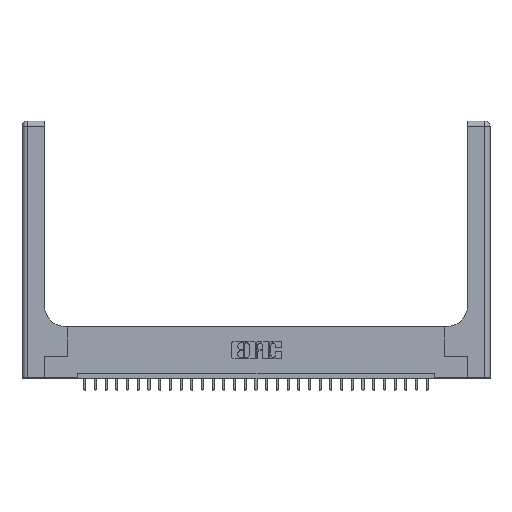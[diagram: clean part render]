
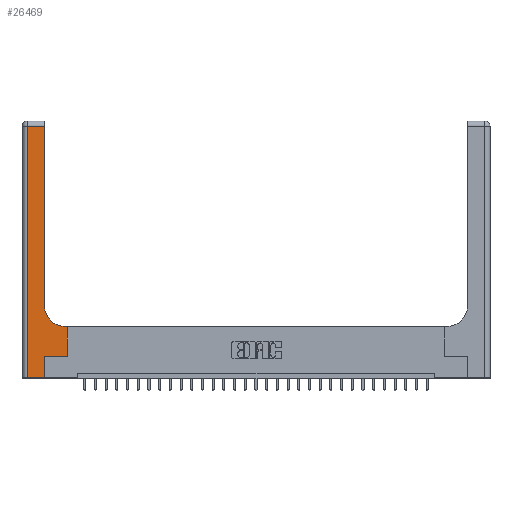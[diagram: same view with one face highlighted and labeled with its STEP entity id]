
A CAD part, top view. The second image highlights one B-rep face of the part: STEP entity #26469.
In plain terms, the highlighted planar face has unit normal (0, 0, 1).
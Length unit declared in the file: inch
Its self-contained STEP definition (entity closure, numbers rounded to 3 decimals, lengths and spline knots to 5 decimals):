
#18 = EDGE_LOOP ( 'NONE', ( #2493, #15372, #7618, #73, #6283, #25855, #7352, #18004, #8994 ) ) ;
#73 = ORIENTED_EDGE ( 'NONE', *, *, #17426, .T. ) ;
#368 = LINE ( 'NONE', #19405, #23107 ) ;
#612 = VERTEX_POINT ( 'NONE', #10977 ) ;
#644 = VECTOR ( 'NONE', #1093, 39.37008 ) ;
#657 = VECTOR ( 'NONE', #3164, 39.37008 ) ;
#1093 = DIRECTION ( 'NONE',  ( 1., 0., 0. ) ) ;
#1325 = CARTESIAN_POINT ( 'NONE',  ( 0.265, 0., 0.37 ) ) ;
#1657 = VERTEX_POINT ( 'NONE', #12036 ) ;
#1805 = VERTEX_POINT ( 'NONE', #18452 ) ;
#1813 = DIRECTION ( 'NONE',  ( 1., 0., 0. ) ) ;
#2021 = EDGE_CURVE ( 'NONE', #4811, #21082, #368, .T. ) ;
#2050 = VECTOR ( 'NONE', #3155, 39.37008 ) ;
#2493 = ORIENTED_EDGE ( 'NONE', *, *, #2021, .T. ) ;
#2524 = CARTESIAN_POINT ( 'NONE',  ( 0., 2.94, 0.37 ) ) ;
#3155 = DIRECTION ( 'NONE',  ( 1., 0., 0. ) ) ;
#3164 = DIRECTION ( 'NONE',  ( 0., 1., 0. ) ) ;
#3475 = EDGE_CURVE ( 'NONE', #21082, #24802, #25972, .T. ) ;
#3976 = CARTESIAN_POINT ( 'NONE',  ( 0.06, 3., 0.37 ) ) ;
#4811 = VERTEX_POINT ( 'NONE', #6078 ) ;
#4902 = EDGE_CURVE ( 'NONE', #612, #4811, #15092, .T. ) ;
#5114 = CARTESIAN_POINT ( 'NONE',  ( 0.265, 0.25, 0.37 ) ) ;
#5139 = DIRECTION ( 'NONE',  ( 0., 1., 0. ) ) ;
#5498 = DIRECTION ( 'NONE',  ( -1., 0., 0. ) ) ;
#5923 = CARTESIAN_POINT ( 'NONE',  ( 0.51, 0.85, 0.37 ) ) ;
#5949 = FACE_OUTER_BOUND ( 'NONE', #18, .T. ) ;
#6078 = CARTESIAN_POINT ( 'NONE',  ( 0.26, 0.85, 0.37 ) ) ;
#6159 = CARTESIAN_POINT ( 'NONE',  ( 0.26, 2.94, 0.37 ) ) ;
#6283 = ORIENTED_EDGE ( 'NONE', *, *, #12287, .T. ) ;
#7228 = EDGE_CURVE ( 'NONE', #22148, #25011, #16596, .T. ) ;
#7295 = VERTEX_POINT ( 'NONE', #7666 ) ;
#7352 = ORIENTED_EDGE ( 'NONE', *, *, #18931, .T. ) ;
#7447 = LINE ( 'NONE', #26327, #15210 ) ;
#7618 = ORIENTED_EDGE ( 'NONE', *, *, #9014, .T. ) ;
#7666 = CARTESIAN_POINT ( 'NONE',  ( 0.265, 0., 0.37 ) ) ;
#7785 = CARTESIAN_POINT ( 'NONE',  ( 0., 3., 0.37 ) ) ;
#8489 = AXIS2_PLACEMENT_3D ( 'NONE', #7785, #26415, #19866 ) ;
#8994 = ORIENTED_EDGE ( 'NONE', *, *, #4902, .T. ) ;
#9014 = EDGE_CURVE ( 'NONE', #24802, #1657, #15174, .T. ) ;
#9021 = CARTESIAN_POINT ( 'NONE',  ( 0.265, 0.25, 0.37 ) ) ;
#9336 = DIRECTION ( 'NONE',  ( 0., 1., 0. ) ) ;
#9707 = CARTESIAN_POINT ( 'NONE',  ( 0.06, 2.94, 0.37 ) ) ;
#10019 = DIRECTION ( 'NONE',  ( 0., 0., -1. ) ) ;
#10115 = LINE ( 'NONE', #1325, #657 ) ;
#10923 = AXIS2_PLACEMENT_3D ( 'NONE', #5923, #10019, #1813 ) ;
#10977 = CARTESIAN_POINT ( 'NONE',  ( 0.51, 0.6, 0.37 ) ) ;
#11532 = LINE ( 'NONE', #17179, #25485 ) ;
#12036 = CARTESIAN_POINT ( 'NONE',  ( 0.06, 0., 0.37 ) ) ;
#12287 = EDGE_CURVE ( 'NONE', #7295, #22148, #10115, .T. ) ;
#14150 = EDGE_CURVE ( 'NONE', #1805, #612, #7447, .T. ) ;
#14924 = DIRECTION ( 'NONE',  ( 0., -1., 0. ) ) ;
#15038 = DIRECTION ( 'NONE',  ( -1., 0., 0. ) ) ;
#15092 = CIRCLE ( 'NONE', #10923, 0.25 ) ;
#15174 = LINE ( 'NONE', #3976, #23576 ) ;
#15210 = VECTOR ( 'NONE', #5498, 39.37008 ) ;
#15271 = VECTOR ( 'NONE', #15038, 39.37008 ) ;
#15372 = ORIENTED_EDGE ( 'NONE', *, *, #3475, .T. ) ;
#15568 = CARTESIAN_POINT ( 'NONE',  ( 0., 0., 0.37 ) ) ;
#16596 = LINE ( 'NONE', #9021, #644 ) ;
#17179 = CARTESIAN_POINT ( 'NONE',  ( 0.528, 0.25, 0.37 ) ) ;
#17426 = EDGE_CURVE ( 'NONE', #1657, #7295, #23129, .T. ) ;
#18004 = ORIENTED_EDGE ( 'NONE', *, *, #14150, .T. ) ;
#18452 = CARTESIAN_POINT ( 'NONE',  ( 0.528, 0.6, 0.37 ) ) ;
#18931 = EDGE_CURVE ( 'NONE', #25011, #1805, #11532, .T. ) ;
#19405 = CARTESIAN_POINT ( 'NONE',  ( 0.26, 3., 0.37 ) ) ;
#19866 = DIRECTION ( 'NONE',  ( -1., 0., 0. ) ) ;
#20045 = PLANE ( 'NONE',  #8489 ) ;
#21082 = VERTEX_POINT ( 'NONE', #6159 ) ;
#22148 = VERTEX_POINT ( 'NONE', #5114 ) ;
#23107 = VECTOR ( 'NONE', #5139, 39.37008 ) ;
#23129 = LINE ( 'NONE', #15568, #2050 ) ;
#23576 = VECTOR ( 'NONE', #14924, 39.37008 ) ;
#24603 = CARTESIAN_POINT ( 'NONE',  ( 0.528, 0.25, 0.37 ) ) ;
#24802 = VERTEX_POINT ( 'NONE', #9707 ) ;
#25011 = VERTEX_POINT ( 'NONE', #24603 ) ;
#25485 = VECTOR ( 'NONE', #9336, 39.37008 ) ;
#25855 = ORIENTED_EDGE ( 'NONE', *, *, #7228, .T. ) ;
#25972 = LINE ( 'NONE', #2524, #15271 ) ;
#26327 = CARTESIAN_POINT ( 'NONE',  ( 0.26, 0.6, 0.37 ) ) ;
#26415 = DIRECTION ( 'NONE',  ( 0., 0., -1. ) ) ;
#26469 = ADVANCED_FACE ( 'NONE', ( #5949 ), #20045, .F. ) ;
